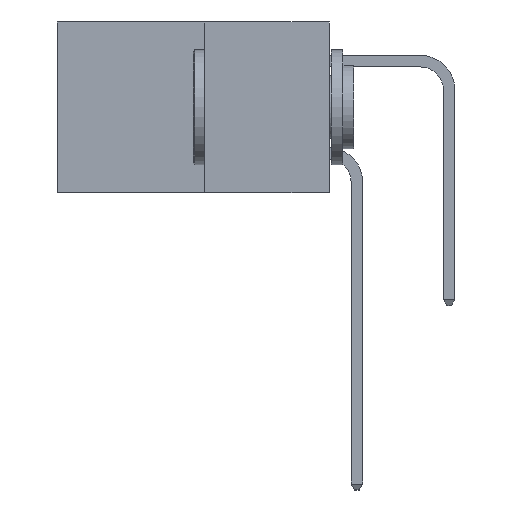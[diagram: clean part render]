
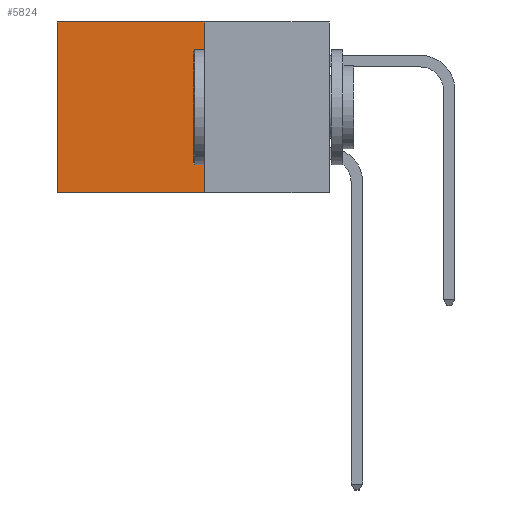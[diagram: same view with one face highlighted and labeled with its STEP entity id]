
A CAD part, left-side view. The second image highlights one B-rep face of the part: STEP entity #5824.
In plain terms, the highlighted planar face has unit normal (-1, 0, 0).
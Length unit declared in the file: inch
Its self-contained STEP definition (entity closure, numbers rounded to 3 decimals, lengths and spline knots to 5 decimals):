
#123 = EDGE_LOOP ( 'NONE', ( #2735, #2671, #2416, #2628 ) ) ;
#444 = LINE ( 'NONE', #7248, #4859 ) ;
#1305 = DIRECTION ( 'NONE',  ( 0., 0., -1. ) ) ;
#1547 = EDGE_CURVE ( 'NONE', #3720, #3676, #4242, .T. ) ;
#2352 = CARTESIAN_POINT ( 'NONE',  ( 0.277, 0.27, 0. ) ) ;
#2416 = ORIENTED_EDGE ( 'NONE', *, *, #9182, .F. ) ;
#2628 = ORIENTED_EDGE ( 'NONE', *, *, #1547, .T. ) ;
#2671 = ORIENTED_EDGE ( 'NONE', *, *, #8178, .F. ) ;
#2735 = ORIENTED_EDGE ( 'NONE', *, *, #8874, .T. ) ;
#2835 = VERTEX_POINT ( 'NONE', #9172 ) ;
#3183 = AXIS2_PLACEMENT_3D ( 'NONE', #4852, #10462, #5742 ) ;
#3374 = CARTESIAN_POINT ( 'NONE',  ( 0.277, 0.27, -0.37 ) ) ;
#3511 = CARTESIAN_POINT ( 'NONE',  ( 0.277, 0.59, 0. ) ) ;
#3584 = LINE ( 'NONE', #8506, #7700 ) ;
#3609 = DIRECTION ( 'NONE',  ( 0., 0., -1. ) ) ;
#3676 = VERTEX_POINT ( 'NONE', #3511 ) ;
#3720 = VERTEX_POINT ( 'NONE', #2352 ) ;
#4161 = CARTESIAN_POINT ( 'NONE',  ( 0.277, 0.27, -0.37 ) ) ;
#4242 = LINE ( 'NONE', #8397, #6480 ) ;
#4810 = PLANE ( 'NONE',  #3183 ) ;
#4852 = CARTESIAN_POINT ( 'NONE',  ( 0.277, 0.27, -0.37 ) ) ;
#4859 = VECTOR ( 'NONE', #1305, 39.37008 ) ;
#4880 = VECTOR ( 'NONE', #6741, 39.37008 ) ;
#5742 = DIRECTION ( 'NONE',  ( 0., 0., -1. ) ) ;
#5824 = ADVANCED_FACE ( 'NONE', ( #7619 ), #4810, .F. ) ;
#6480 = VECTOR ( 'NONE', #8816, 39.37008 ) ;
#6741 = DIRECTION ( 'NONE',  ( 0., 1., 0. ) ) ;
#7248 = CARTESIAN_POINT ( 'NONE',  ( 0.277, 0.27, -0.37 ) ) ;
#7588 = VERTEX_POINT ( 'NONE', #4161 ) ;
#7619 = FACE_OUTER_BOUND ( 'NONE', #123, .T. ) ;
#7700 = VECTOR ( 'NONE', #3609, 39.37008 ) ;
#8178 = EDGE_CURVE ( 'NONE', #7588, #2835, #9184, .T. ) ;
#8397 = CARTESIAN_POINT ( 'NONE',  ( 0.277, 0.27, 0. ) ) ;
#8506 = CARTESIAN_POINT ( 'NONE',  ( 0.277, 0.59, -0.37 ) ) ;
#8816 = DIRECTION ( 'NONE',  ( 0., 1., 0. ) ) ;
#8874 = EDGE_CURVE ( 'NONE', #3676, #2835, #3584, .T. ) ;
#9172 = CARTESIAN_POINT ( 'NONE',  ( 0.277, 0.59, -0.37 ) ) ;
#9182 = EDGE_CURVE ( 'NONE', #3720, #7588, #444, .T. ) ;
#9184 = LINE ( 'NONE', #3374, #4880 ) ;
#10462 = DIRECTION ( 'NONE',  ( 1., 0., 0. ) ) ;
